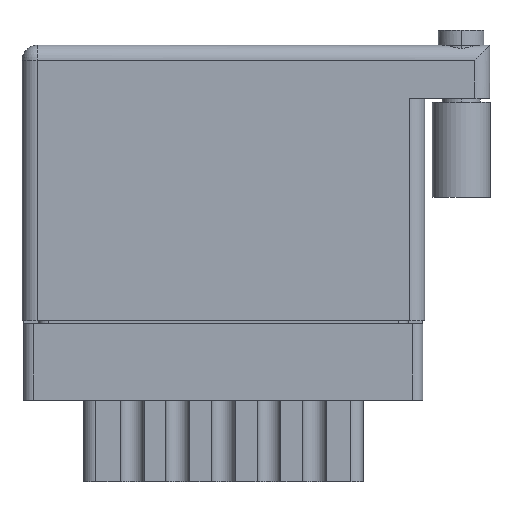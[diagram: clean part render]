
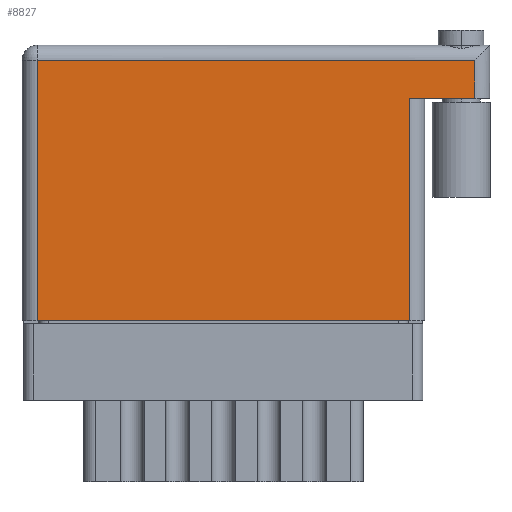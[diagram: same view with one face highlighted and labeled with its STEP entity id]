
A CAD part, front view. The second image highlights one B-rep face of the part: STEP entity #8827.
In plain terms, the highlighted face is planar.
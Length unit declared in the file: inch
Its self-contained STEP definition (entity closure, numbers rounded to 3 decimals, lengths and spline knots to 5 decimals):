
#65 = VERTEX_POINT ( 'NONE', #7089 ) ;
#663 = DIRECTION ( 'NONE',  ( 0., -1., 0. ) ) ;
#1219 = DIRECTION ( 'NONE',  ( -1., 0., 0. ) ) ;
#2037 = DIRECTION ( 'NONE',  ( 0., 1., 0. ) ) ;
#2760 = CARTESIAN_POINT ( 'NONE',  ( 0.05, 0., 0. ) ) ;
#3045 = EDGE_CURVE ( 'NONE', #5864, #8644, #9045, .T. ) ;
#3237 = CARTESIAN_POINT ( 'NONE',  ( 1.275, 0., 0. ) ) ;
#3489 = VECTOR ( 'NONE', #2037, 39.37008 ) ;
#4107 = ORIENTED_EDGE ( 'NONE', *, *, #25888, .T. ) ;
#4851 = CARTESIAN_POINT ( 'NONE',  ( 1.489, 0.856, 0. ) ) ;
#5864 = VERTEX_POINT ( 'NONE', #3237 ) ;
#6038 = EDGE_CURVE ( 'NONE', #8594, #15133, #19739, .T. ) ;
#6083 = VECTOR ( 'NONE', #14894, 39.37008 ) ;
#6799 = ORIENTED_EDGE ( 'NONE', *, *, #3045, .T. ) ;
#6830 = DIRECTION ( 'NONE',  ( 0., 0., -1. ) ) ;
#6870 = DIRECTION ( 'NONE',  ( -1., 0., 0. ) ) ;
#7089 = CARTESIAN_POINT ( 'NONE',  ( 0.05, 0., 0. ) ) ;
#8594 = VERTEX_POINT ( 'NONE', #4851 ) ;
#8644 = VERTEX_POINT ( 'NONE', #25546 ) ;
#8827 = ADVANCED_FACE ( 'NONE', ( #23579 ), #17642, .F. ) ;
#9045 = LINE ( 'NONE', #12444, #3489 ) ;
#9074 = CARTESIAN_POINT ( 'NONE',  ( 0., 0., 0. ) ) ;
#9114 = CARTESIAN_POINT ( 'NONE',  ( 0., 0.906, 0. ) ) ;
#11263 = ORIENTED_EDGE ( 'NONE', *, *, #25717, .T. ) ;
#12075 = VERTEX_POINT ( 'NONE', #21719 ) ;
#12444 = CARTESIAN_POINT ( 'NONE',  ( 1.275, 0.731, 0. ) ) ;
#13280 = LINE ( 'NONE', #27073, #6083 ) ;
#13300 = EDGE_CURVE ( 'NONE', #65, #5864, #23899, .T. ) ;
#13440 = CARTESIAN_POINT ( 'NONE',  ( 0.05, 0.856, 0. ) ) ;
#14070 = AXIS2_PLACEMENT_3D ( 'NONE', #9114, #6830, #26080 ) ;
#14481 = LINE ( 'NONE', #17410, #18456 ) ;
#14709 = ORIENTED_EDGE ( 'NONE', *, *, #24294, .F. ) ;
#14894 = DIRECTION ( 'NONE',  ( 0., 1., 0. ) ) ;
#15133 = VERTEX_POINT ( 'NONE', #13440 ) ;
#15286 = DIRECTION ( 'NONE',  ( 1., 0., 0. ) ) ;
#15903 = VECTOR ( 'NONE', #663, 39.37008 ) ;
#17225 = LINE ( 'NONE', #2760, #15903 ) ;
#17410 = CARTESIAN_POINT ( 'NONE',  ( 1.539, 0.731, 0. ) ) ;
#17642 = PLANE ( 'NONE',  #14070 ) ;
#18456 = VECTOR ( 'NONE', #6870, 39.37008 ) ;
#19739 = LINE ( 'NONE', #20176, #21388 ) ;
#20176 = CARTESIAN_POINT ( 'NONE',  ( 0., 0.856, 0. ) ) ;
#21388 = VECTOR ( 'NONE', #1219, 39.37008 ) ;
#21719 = CARTESIAN_POINT ( 'NONE',  ( 1.489, 0.731, 0. ) ) ;
#23533 = ORIENTED_EDGE ( 'NONE', *, *, #13300, .T. ) ;
#23579 = FACE_OUTER_BOUND ( 'NONE', #26146, .T. ) ;
#23783 = ORIENTED_EDGE ( 'NONE', *, *, #6038, .T. ) ;
#23899 = LINE ( 'NONE', #9074, #26872 ) ;
#24294 = EDGE_CURVE ( 'NONE', #12075, #8644, #14481, .T. ) ;
#25546 = CARTESIAN_POINT ( 'NONE',  ( 1.275, 0.731, 0. ) ) ;
#25717 = EDGE_CURVE ( 'NONE', #12075, #8594, #13280, .T. ) ;
#25888 = EDGE_CURVE ( 'NONE', #15133, #65, #17225, .T. ) ;
#26080 = DIRECTION ( 'NONE',  ( -1., 0., 0. ) ) ;
#26146 = EDGE_LOOP ( 'NONE', ( #23533, #6799, #14709, #11263, #23783, #4107 ) ) ;
#26872 = VECTOR ( 'NONE', #15286, 39.37008 ) ;
#27073 = CARTESIAN_POINT ( 'NONE',  ( 1.489, 0.906, 0. ) ) ;
